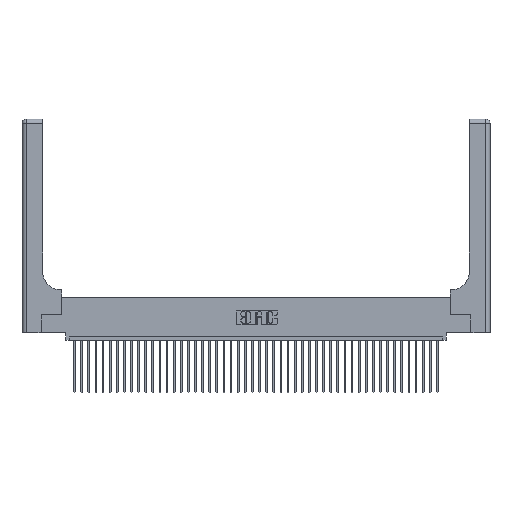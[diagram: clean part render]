
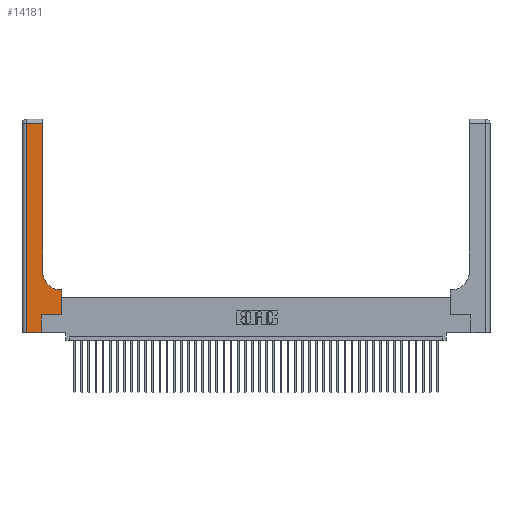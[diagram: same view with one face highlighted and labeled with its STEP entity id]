
A CAD part, top view. The second image highlights one B-rep face of the part: STEP entity #14181.
In plain terms, the highlighted planar face has unit normal (0, 0, 1).
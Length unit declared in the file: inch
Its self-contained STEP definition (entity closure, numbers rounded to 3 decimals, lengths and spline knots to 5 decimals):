
#433 = VERTEX_POINT ( 'NONE', #21546 ) ;
#1322 = ORIENTED_EDGE ( 'NONE', *, *, #13922, .T. ) ;
#1527 = LINE ( 'NONE', #3577, #18664 ) ;
#2959 = LINE ( 'NONE', #22393, #32606 ) ;
#2990 = AXIS2_PLACEMENT_3D ( 'NONE', #22654, #28769, #8891 ) ;
#3201 = CARTESIAN_POINT ( 'NONE',  ( 0.5415, 0.85, 0.37 ) ) ;
#3385 = VECTOR ( 'NONE', #24060, 39.37008 ) ;
#3577 = CARTESIAN_POINT ( 'NONE',  ( 0.5585, 0.25, 0.37 ) ) ;
#3620 = CARTESIAN_POINT ( 'NONE',  ( 0.06, 2.94, 0.37 ) ) ;
#4127 = DIRECTION ( 'NONE',  ( 0., -1., 0. ) ) ;
#4540 = LINE ( 'NONE', #20638, #27822 ) ;
#6183 = FACE_OUTER_BOUND ( 'NONE', #40390, .T. ) ;
#7203 = AXIS2_PLACEMENT_3D ( 'NONE', #3201, #23250, #16377 ) ;
#7399 = VECTOR ( 'NONE', #27931, 39.37008 ) ;
#7518 = CARTESIAN_POINT ( 'NONE',  ( 0.269, 0.25, 0.37 ) ) ;
#7670 = EDGE_CURVE ( 'NONE', #12952, #25506, #4540, .T. ) ;
#7769 = EDGE_CURVE ( 'NONE', #25652, #35560, #33886, .T. ) ;
#8174 = LINE ( 'NONE', #22320, #13840 ) ;
#8689 = CARTESIAN_POINT ( 'NONE',  ( 0.5415, 0.6, 0.37 ) ) ;
#8891 = DIRECTION ( 'NONE',  ( -1., 0., 0. ) ) ;
#9058 = DIRECTION ( 'NONE',  ( -1., 0., 0. ) ) ;
#11698 = DIRECTION ( 'NONE',  ( 1., 0., 0. ) ) ;
#12356 = VERTEX_POINT ( 'NONE', #37812 ) ;
#12572 = DIRECTION ( 'NONE',  ( 0., 1., 0. ) ) ;
#12717 = VERTEX_POINT ( 'NONE', #30734 ) ;
#12763 = ORIENTED_EDGE ( 'NONE', *, *, #14876, .T. ) ;
#12808 = EDGE_CURVE ( 'NONE', #25506, #18313, #19393, .T. ) ;
#12952 = VERTEX_POINT ( 'NONE', #3620 ) ;
#12957 = ORIENTED_EDGE ( 'NONE', *, *, #31833, .T. ) ;
#13788 = ORIENTED_EDGE ( 'NONE', *, *, #12808, .T. ) ;
#13840 = VECTOR ( 'NONE', #12572, 39.37008 ) ;
#13873 = VERTEX_POINT ( 'NONE', #27787 ) ;
#13922 = EDGE_CURVE ( 'NONE', #35560, #13873, #28450, .T. ) ;
#14181 = ADVANCED_FACE ( 'NONE', ( #6183 ), #18141, .F. ) ;
#14876 = EDGE_CURVE ( 'NONE', #18313, #433, #2959, .T. ) ;
#16377 = DIRECTION ( 'NONE',  ( 1., 0., 0. ) ) ;
#18141 = PLANE ( 'NONE',  #2990 ) ;
#18313 = VERTEX_POINT ( 'NONE', #23446 ) ;
#18664 = VECTOR ( 'NONE', #36286, 39.37008 ) ;
#19393 = LINE ( 'NONE', #31464, #40252 ) ;
#20638 = CARTESIAN_POINT ( 'NONE',  ( 0.06, 3., 0.37 ) ) ;
#21546 = CARTESIAN_POINT ( 'NONE',  ( 0.269, 0.25, 0.37 ) ) ;
#21744 = EDGE_CURVE ( 'NONE', #12356, #25652, #1527, .T. ) ;
#22320 = CARTESIAN_POINT ( 'NONE',  ( 0.2915, 3., 0.37 ) ) ;
#22393 = CARTESIAN_POINT ( 'NONE',  ( 0.269, 0., 0.37 ) ) ;
#22654 = CARTESIAN_POINT ( 'NONE',  ( 0., 3., 0.37 ) ) ;
#22811 = ORIENTED_EDGE ( 'NONE', *, *, #21744, .T. ) ;
#23250 = DIRECTION ( 'NONE',  ( 0., 0., -1. ) ) ;
#23446 = CARTESIAN_POINT ( 'NONE',  ( 0.269, 0., 0.37 ) ) ;
#24060 = DIRECTION ( 'NONE',  ( 1., 0., 0. ) ) ;
#25506 = VERTEX_POINT ( 'NONE', #36080 ) ;
#25652 = VERTEX_POINT ( 'NONE', #41563 ) ;
#25761 = DIRECTION ( 'NONE',  ( 0., 1., 0. ) ) ;
#26840 = ORIENTED_EDGE ( 'NONE', *, *, #31699, .T. ) ;
#27324 = LINE ( 'NONE', #7518, #3385 ) ;
#27787 = CARTESIAN_POINT ( 'NONE',  ( 0.2915, 0.85, 0.37 ) ) ;
#27822 = VECTOR ( 'NONE', #4127, 39.37008 ) ;
#27931 = DIRECTION ( 'NONE',  ( -1., 0., 0. ) ) ;
#28450 = CIRCLE ( 'NONE', #7203, 0.25 ) ;
#28769 = DIRECTION ( 'NONE',  ( 0., 0., -1. ) ) ;
#30734 = CARTESIAN_POINT ( 'NONE',  ( 0.2915, 2.94, 0.37 ) ) ;
#31464 = CARTESIAN_POINT ( 'NONE',  ( 0., 0., 0.37 ) ) ;
#31699 = EDGE_CURVE ( 'NONE', #12717, #12952, #36208, .T. ) ;
#31833 = EDGE_CURVE ( 'NONE', #13873, #12717, #8174, .T. ) ;
#32472 = EDGE_CURVE ( 'NONE', #433, #12356, #27324, .T. ) ;
#32606 = VECTOR ( 'NONE', #25761, 39.37008 ) ;
#33886 = LINE ( 'NONE', #35191, #7399 ) ;
#35191 = CARTESIAN_POINT ( 'NONE',  ( 0.2915, 0.6, 0.37 ) ) ;
#35488 = CARTESIAN_POINT ( 'NONE',  ( 0., 2.94, 0.37 ) ) ;
#35560 = VERTEX_POINT ( 'NONE', #8689 ) ;
#35701 = VECTOR ( 'NONE', #9058, 39.37008 ) ;
#36080 = CARTESIAN_POINT ( 'NONE',  ( 0.06, 0., 0.37 ) ) ;
#36208 = LINE ( 'NONE', #35488, #35701 ) ;
#36286 = DIRECTION ( 'NONE',  ( 0., 1., 0. ) ) ;
#36399 = ORIENTED_EDGE ( 'NONE', *, *, #32472, .T. ) ;
#37812 = CARTESIAN_POINT ( 'NONE',  ( 0.5585, 0.25, 0.37 ) ) ;
#38339 = ORIENTED_EDGE ( 'NONE', *, *, #7769, .T. ) ;
#40252 = VECTOR ( 'NONE', #11698, 39.37008 ) ;
#40390 = EDGE_LOOP ( 'NONE', ( #12957, #26840, #41997, #13788, #12763, #36399, #22811, #38339, #1322 ) ) ;
#41563 = CARTESIAN_POINT ( 'NONE',  ( 0.5585, 0.6, 0.37 ) ) ;
#41997 = ORIENTED_EDGE ( 'NONE', *, *, #7670, .T. ) ;
